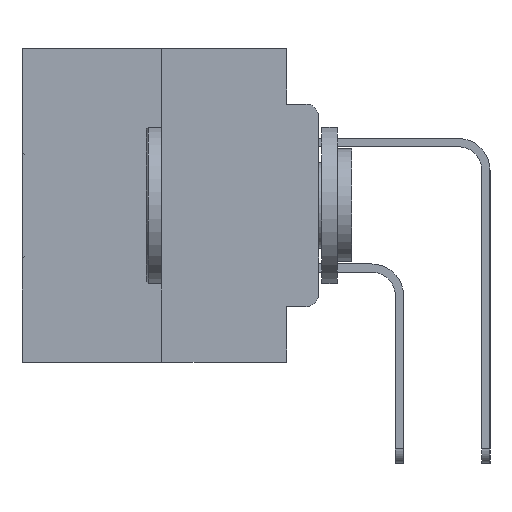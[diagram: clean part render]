
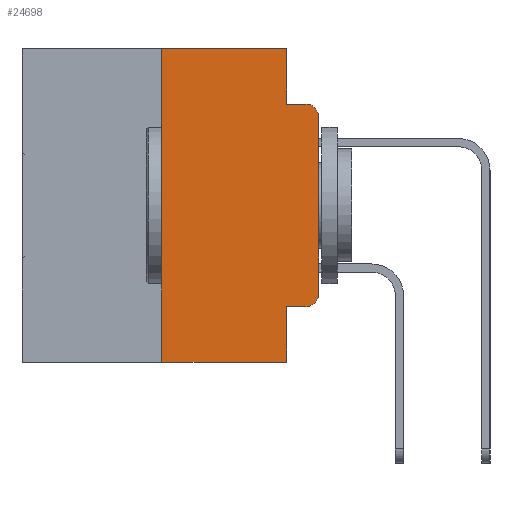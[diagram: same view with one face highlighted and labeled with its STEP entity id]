
A CAD part, left-side view. The second image highlights one B-rep face of the part: STEP entity #24698.
In plain terms, the highlighted planar face has unit normal (-1, 0, 0).
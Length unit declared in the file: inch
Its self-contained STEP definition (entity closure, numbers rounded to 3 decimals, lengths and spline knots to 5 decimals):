
#690 = CARTESIAN_POINT ( 'NONE',  ( 0., 0.473, -0.5 ) ) ;
#2278 = DIRECTION ( 'NONE',  ( -1., 0., 0. ) ) ;
#2564 = CARTESIAN_POINT ( 'NONE',  ( 0., 0.25, 0. ) ) ;
#2923 = ORIENTED_EDGE ( 'NONE', *, *, #20369, .F. ) ;
#3110 = CARTESIAN_POINT ( 'NONE',  ( 0., 0.051, 0. ) ) ;
#3112 = DIRECTION ( 'NONE',  ( 0., -1., 0. ) ) ;
#3148 = EDGE_CURVE ( 'NONE', #9011, #27531, #31528, .T. ) ;
#3693 = CARTESIAN_POINT ( 'NONE',  ( 0., 0.051, -0.4115 ) ) ;
#4074 = ORIENTED_EDGE ( 'NONE', *, *, #4299, .T. ) ;
#4091 = CARTESIAN_POINT ( 'NONE',  ( 0., 0.051, 0. ) ) ;
#4299 = EDGE_CURVE ( 'NONE', #18995, #18149, #18124, .T. ) ;
#4361 = CIRCLE ( 'NONE', #8272, 0.02 ) ;
#4430 = ORIENTED_EDGE ( 'NONE', *, *, #19214, .F. ) ;
#4510 = CARTESIAN_POINT ( 'NONE',  ( 0., 0., -0.3915 ) ) ;
#4607 = LINE ( 'NONE', #22837, #29328 ) ;
#4797 = EDGE_CURVE ( 'NONE', #18995, #5540, #24474, .T. ) ;
#5303 = VECTOR ( 'NONE', #8549, 39.37008 ) ;
#5540 = VERTEX_POINT ( 'NONE', #25193 ) ;
#5586 = ORIENTED_EDGE ( 'NONE', *, *, #3148, .T. ) ;
#5829 = LINE ( 'NONE', #23453, #6622 ) ;
#6047 = CARTESIAN_POINT ( 'NONE',  ( 0., 0.051, -0.4115 ) ) ;
#6375 = CARTESIAN_POINT ( 'NONE',  ( 0., 0.473, 0. ) ) ;
#6508 = VECTOR ( 'NONE', #8680, 39.37008 ) ;
#6556 = DIRECTION ( 'NONE',  ( 0., 0., -1. ) ) ;
#6622 = VECTOR ( 'NONE', #8552, 39.37008 ) ;
#8272 = AXIS2_PLACEMENT_3D ( 'NONE', #17104, #2278, #19588 ) ;
#8277 = ORIENTED_EDGE ( 'NONE', *, *, #31601, .T. ) ;
#8549 = DIRECTION ( 'NONE',  ( 0., -1., 0. ) ) ;
#8552 = DIRECTION ( 'NONE',  ( 0., -1., 0. ) ) ;
#8680 = DIRECTION ( 'NONE',  ( 0., -1., 0. ) ) ;
#8894 = CARTESIAN_POINT ( 'NONE',  ( 0., 0.02, -0.3915 ) ) ;
#9011 = VERTEX_POINT ( 'NONE', #3693 ) ;
#9050 = FACE_OUTER_BOUND ( 'NONE', #16395, .T. ) ;
#9231 = VERTEX_POINT ( 'NONE', #4510 ) ;
#10207 = CARTESIAN_POINT ( 'NONE',  ( 0., 0.25, -0.5 ) ) ;
#10973 = VERTEX_POINT ( 'NONE', #28399 ) ;
#11384 = DIRECTION ( 'NONE',  ( 1., 0., 0. ) ) ;
#11398 = DIRECTION ( 'NONE',  ( 0., 0., -1. ) ) ;
#11845 = ORIENTED_EDGE ( 'NONE', *, *, #26817, .T. ) ;
#11950 = DIRECTION ( 'NONE',  ( 0., 0., 1. ) ) ;
#12653 = VERTEX_POINT ( 'NONE', #31215 ) ;
#12973 = DIRECTION ( 'NONE',  ( 0., 0., -1. ) ) ;
#13089 = AXIS2_PLACEMENT_3D ( 'NONE', #6375, #11384, #28625 ) ;
#13993 = VERTEX_POINT ( 'NONE', #31674 ) ;
#16395 = EDGE_LOOP ( 'NONE', ( #20726, #8277, #16483, #2923, #4430, #23091, #4074, #18091, #5586, #11845 ) ) ;
#16483 = ORIENTED_EDGE ( 'NONE', *, *, #28565, .F. ) ;
#17104 = CARTESIAN_POINT ( 'NONE',  ( 0., 0.02, -0.1085 ) ) ;
#17513 = EDGE_CURVE ( 'NONE', #9231, #12653, #29178, .T. ) ;
#17957 = VECTOR ( 'NONE', #24817, 39.37008 ) ;
#18091 = ORIENTED_EDGE ( 'NONE', *, *, #25347, .F. ) ;
#18124 = LINE ( 'NONE', #690, #29546 ) ;
#18149 = VERTEX_POINT ( 'NONE', #21548 ) ;
#18995 = VERTEX_POINT ( 'NONE', #10207 ) ;
#19214 = EDGE_CURVE ( 'NONE', #5540, #20936, #5829, .T. ) ;
#19588 = DIRECTION ( 'NONE',  ( 0., 0., -1. ) ) ;
#20369 = EDGE_CURVE ( 'NONE', #20936, #13993, #4607, .T. ) ;
#20726 = ORIENTED_EDGE ( 'NONE', *, *, #17513, .T. ) ;
#20936 = VERTEX_POINT ( 'NONE', #3110 ) ;
#21548 = CARTESIAN_POINT ( 'NONE',  ( 0., 0.051, -0.5 ) ) ;
#22837 = CARTESIAN_POINT ( 'NONE',  ( 0., 0.051, 0. ) ) ;
#23091 = ORIENTED_EDGE ( 'NONE', *, *, #4797, .F. ) ;
#23453 = CARTESIAN_POINT ( 'NONE',  ( 0., 0.473, 0. ) ) ;
#23832 = VECTOR ( 'NONE', #6556, 39.37008 ) ;
#24474 = LINE ( 'NONE', #2564, #17957 ) ;
#24698 = ADVANCED_FACE ( 'NONE', ( #9050 ), #26094, .F. ) ;
#24817 = DIRECTION ( 'NONE',  ( 0., 0., 1. ) ) ;
#25193 = CARTESIAN_POINT ( 'NONE',  ( 0., 0.25, 0. ) ) ;
#25347 = EDGE_CURVE ( 'NONE', #9011, #18149, #31765, .T. ) ;
#25627 = CIRCLE ( 'NONE', #26968, 0.02 ) ;
#26094 = PLANE ( 'NONE',  #13089 ) ;
#26213 = DIRECTION ( 'NONE',  ( -1., 0., 0. ) ) ;
#26817 = EDGE_CURVE ( 'NONE', #27531, #9231, #25627, .T. ) ;
#26830 = CARTESIAN_POINT ( 'NONE',  ( 0., 0.02, -0.4115 ) ) ;
#26968 = AXIS2_PLACEMENT_3D ( 'NONE', #8894, #26213, #11398 ) ;
#27037 = LINE ( 'NONE', #28447, #6508 ) ;
#27531 = VERTEX_POINT ( 'NONE', #26830 ) ;
#28399 = CARTESIAN_POINT ( 'NONE',  ( 0., 0.02, -0.0885 ) ) ;
#28447 = CARTESIAN_POINT ( 'NONE',  ( 0., 0.051, -0.0885 ) ) ;
#28565 = EDGE_CURVE ( 'NONE', #13993, #10973, #27037, .T. ) ;
#28625 = DIRECTION ( 'NONE',  ( 0., 0., -1. ) ) ;
#29178 = LINE ( 'NONE', #31588, #31392 ) ;
#29328 = VECTOR ( 'NONE', #12973, 39.37008 ) ;
#29546 = VECTOR ( 'NONE', #3112, 39.37008 ) ;
#31215 = CARTESIAN_POINT ( 'NONE',  ( 0., 0., -0.1085 ) ) ;
#31392 = VECTOR ( 'NONE', #11950, 39.37008 ) ;
#31528 = LINE ( 'NONE', #6047, #5303 ) ;
#31588 = CARTESIAN_POINT ( 'NONE',  ( 0., 0., 0. ) ) ;
#31601 = EDGE_CURVE ( 'NONE', #12653, #10973, #4361, .T. ) ;
#31674 = CARTESIAN_POINT ( 'NONE',  ( 0., 0.051, -0.0885 ) ) ;
#31765 = LINE ( 'NONE', #4091, #23832 ) ;
